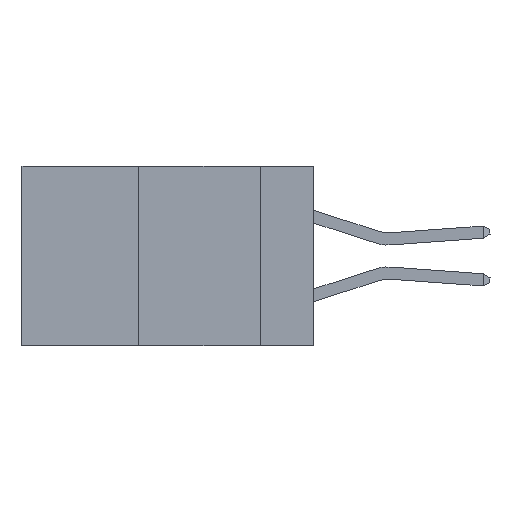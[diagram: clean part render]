
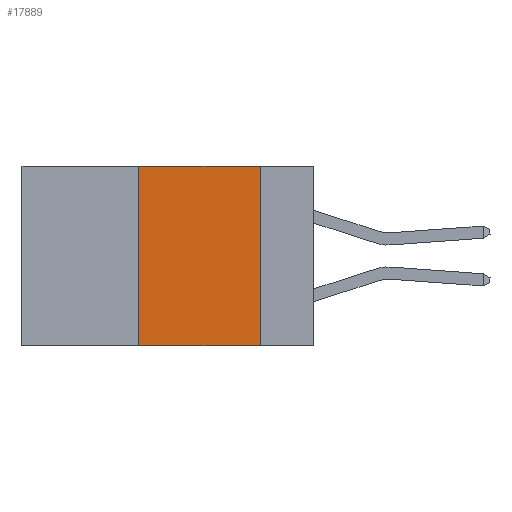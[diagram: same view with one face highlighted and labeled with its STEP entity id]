
A CAD part, left-side view. The second image highlights one B-rep face of the part: STEP entity #17889.
In plain terms, the highlighted planar face has unit normal (-1, 0, 0).
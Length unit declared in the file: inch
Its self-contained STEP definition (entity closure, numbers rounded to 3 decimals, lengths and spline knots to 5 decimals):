
#344 = ORIENTED_EDGE ( 'NONE', *, *, #8215, .T. ) ;
#464 = DIRECTION ( 'NONE',  ( 0., -1., 0. ) ) ;
#617 = DIRECTION ( 'NONE',  ( 0., 0., -1. ) ) ;
#794 = CARTESIAN_POINT ( 'NONE',  ( 0., 0.6, -0.37 ) ) ;
#1186 = DIRECTION ( 'NONE',  ( 0., 0., -1. ) ) ;
#1259 = ORIENTED_EDGE ( 'NONE', *, *, #11046, .F. ) ;
#1501 = VECTOR ( 'NONE', #1186, 39.37008 ) ;
#1515 = VECTOR ( 'NONE', #464, 39.37008 ) ;
#2052 = LINE ( 'NONE', #3886, #15678 ) ;
#2462 = ORIENTED_EDGE ( 'NONE', *, *, #15538, .F. ) ;
#2605 = VERTEX_POINT ( 'NONE', #7020 ) ;
#3093 = VERTEX_POINT ( 'NONE', #9897 ) ;
#3886 = CARTESIAN_POINT ( 'NONE',  ( 0., 0.36, 0. ) ) ;
#4591 = VERTEX_POINT ( 'NONE', #12324 ) ;
#4980 = PLANE ( 'NONE',  #15978 ) ;
#5001 = ORIENTED_EDGE ( 'NONE', *, *, #13827, .F. ) ;
#5073 = EDGE_LOOP ( 'NONE', ( #2462, #5001, #1259, #344 ) ) ;
#6471 = CARTESIAN_POINT ( 'NONE',  ( 0., 0.36, -0.37 ) ) ;
#7020 = CARTESIAN_POINT ( 'NONE',  ( 0., 0.11, 0. ) ) ;
#8215 = EDGE_CURVE ( 'NONE', #10188, #3093, #11066, .T. ) ;
#8635 = LINE ( 'NONE', #9766, #1501 ) ;
#9225 = DIRECTION ( 'NONE',  ( 1., 0., 0. ) ) ;
#9766 = CARTESIAN_POINT ( 'NONE',  ( 0., 0.11, 0. ) ) ;
#9897 = CARTESIAN_POINT ( 'NONE',  ( 0., 0.11, -0.37 ) ) ;
#10188 = VERTEX_POINT ( 'NONE', #6471 ) ;
#10515 = CARTESIAN_POINT ( 'NONE',  ( 0., 0.6, 0. ) ) ;
#10765 = DIRECTION ( 'NONE',  ( 0., -1., 0. ) ) ;
#11046 = EDGE_CURVE ( 'NONE', #10188, #4591, #2052, .T. ) ;
#11066 = LINE ( 'NONE', #794, #11921 ) ;
#11921 = VECTOR ( 'NONE', #10765, 39.37008 ) ;
#12324 = CARTESIAN_POINT ( 'NONE',  ( 0., 0.36, 0. ) ) ;
#12379 = LINE ( 'NONE', #10515, #1515 ) ;
#12493 = FACE_OUTER_BOUND ( 'NONE', #5073, .T. ) ;
#13827 = EDGE_CURVE ( 'NONE', #4591, #2605, #12379, .T. ) ;
#15538 = EDGE_CURVE ( 'NONE', #2605, #3093, #8635, .T. ) ;
#15678 = VECTOR ( 'NONE', #16363, 39.37008 ) ;
#15978 = AXIS2_PLACEMENT_3D ( 'NONE', #17461, #9225, #617 ) ;
#16363 = DIRECTION ( 'NONE',  ( 0., 0., 1. ) ) ;
#17461 = CARTESIAN_POINT ( 'NONE',  ( 0., 0.6, 0. ) ) ;
#17889 = ADVANCED_FACE ( 'NONE', ( #12493 ), #4980, .F. ) ;
